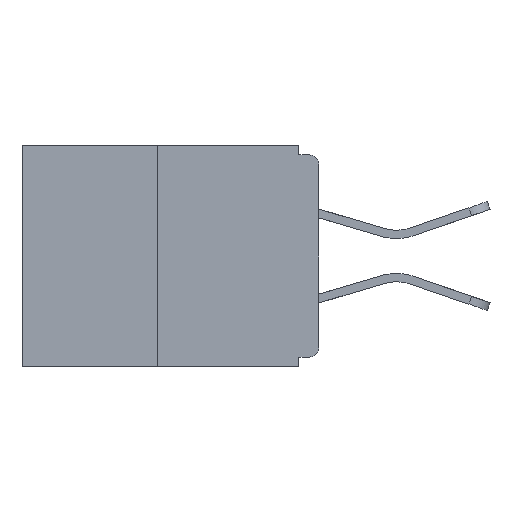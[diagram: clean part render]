
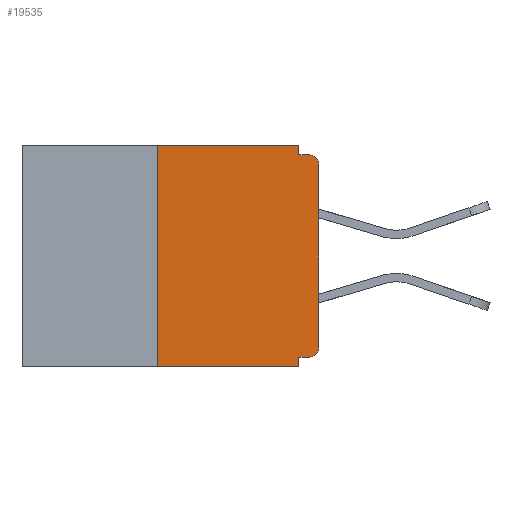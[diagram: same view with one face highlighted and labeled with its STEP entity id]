
A CAD part, left-side view. The second image highlights one B-rep face of the part: STEP entity #19535.
In plain terms, the highlighted planar face has unit normal (-1, 0, 0).
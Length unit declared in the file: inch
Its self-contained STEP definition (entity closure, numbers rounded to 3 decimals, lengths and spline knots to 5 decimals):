
#85 = CARTESIAN_POINT ( 'NONE',  ( 0., 0.015, -0.328 ) ) ;
#91 = LINE ( 'NONE', #1999, #10467 ) ;
#777 = LINE ( 'NONE', #20366, #14387 ) ;
#1901 = CARTESIAN_POINT ( 'NONE',  ( 0., 0., -0.313 ) ) ;
#1999 = CARTESIAN_POINT ( 'NONE',  ( 0., 0., -0.328 ) ) ;
#2536 = CARTESIAN_POINT ( 'NONE',  ( 0., 0.015, -0.015 ) ) ;
#2837 = AXIS2_PLACEMENT_3D ( 'NONE', #25909, #21193, #9138 ) ;
#2928 = DIRECTION ( 'NONE',  ( 0., -1., 0. ) ) ;
#3150 = CARTESIAN_POINT ( 'NONE',  ( 0., 0.031, -0.015 ) ) ;
#4056 = CARTESIAN_POINT ( 'NONE',  ( 0., 0.46, -0.343 ) ) ;
#4239 = DIRECTION ( 'NONE',  ( -1., 0., 0. ) ) ;
#4346 = CARTESIAN_POINT ( 'NONE',  ( 0., 0.015, -0.313 ) ) ;
#4563 = VERTEX_POINT ( 'NONE', #6031 ) ;
#4624 = ORIENTED_EDGE ( 'NONE', *, *, #10382, .F. ) ;
#5428 = EDGE_CURVE ( 'NONE', #14202, #19848, #8894, .T. ) ;
#5958 = EDGE_LOOP ( 'NONE', ( #14963, #21630, #27414, #29288, #4624, #13181, #27754, #19563, #12750, #11808 ) ) ;
#6020 = VECTOR ( 'NONE', #15183, 39.37008 ) ;
#6031 = CARTESIAN_POINT ( 'NONE',  ( 0., 0.25, 0. ) ) ;
#6893 = VERTEX_POINT ( 'NONE', #2536 ) ;
#7083 = VERTEX_POINT ( 'NONE', #10704 ) ;
#7120 = VERTEX_POINT ( 'NONE', #1901 ) ;
#7920 = DIRECTION ( 'NONE',  ( 0., 0., -1. ) ) ;
#8058 = EDGE_CURVE ( 'NONE', #12188, #31089, #14869, .T. ) ;
#8218 = CARTESIAN_POINT ( 'NONE',  ( 0., 0., 0. ) ) ;
#8294 = DIRECTION ( 'NONE',  ( 0., 0., -1. ) ) ;
#8894 = LINE ( 'NONE', #4056, #10368 ) ;
#9138 = DIRECTION ( 'NONE',  ( 0., 0., -1. ) ) ;
#9145 = EDGE_CURVE ( 'NONE', #4563, #12188, #777, .T. ) ;
#9616 = LINE ( 'NONE', #29054, #30650 ) ;
#10024 = CARTESIAN_POINT ( 'NONE',  ( 0., 0.031, -0.343 ) ) ;
#10355 = DIRECTION ( 'NONE',  ( 0., -1., 0. ) ) ;
#10368 = VECTOR ( 'NONE', #25677, 39.37008 ) ;
#10382 = EDGE_CURVE ( 'NONE', #16863, #7083, #91, .T. ) ;
#10456 = AXIS2_PLACEMENT_3D ( 'NONE', #13997, #4239, #21135 ) ;
#10467 = VECTOR ( 'NONE', #31000, 39.37008 ) ;
#10704 = CARTESIAN_POINT ( 'NONE',  ( 0., 0.031, -0.328 ) ) ;
#10972 = CIRCLE ( 'NONE', #10456, 0.015 ) ;
#11144 = AXIS2_PLACEMENT_3D ( 'NONE', #4346, #18560, #18248 ) ;
#11808 = ORIENTED_EDGE ( 'NONE', *, *, #8058, .F. ) ;
#12188 = VERTEX_POINT ( 'NONE', #18408 ) ;
#12449 = DIRECTION ( 'NONE',  ( 0., 0., 1. ) ) ;
#12750 = ORIENTED_EDGE ( 'NONE', *, *, #18966, .F. ) ;
#13181 = ORIENTED_EDGE ( 'NONE', *, *, #30544, .T. ) ;
#13997 = CARTESIAN_POINT ( 'NONE',  ( 0., 0.015, -0.03 ) ) ;
#14202 = VERTEX_POINT ( 'NONE', #30343 ) ;
#14387 = VECTOR ( 'NONE', #10355, 39.37008 ) ;
#14869 = LINE ( 'NONE', #29579, #15141 ) ;
#14963 = ORIENTED_EDGE ( 'NONE', *, *, #9145, .F. ) ;
#15141 = VECTOR ( 'NONE', #7920, 39.37008 ) ;
#15183 = DIRECTION ( 'NONE',  ( 0., 0., 1. ) ) ;
#15695 = CIRCLE ( 'NONE', #11144, 0.015 ) ;
#16863 = VERTEX_POINT ( 'NONE', #85 ) ;
#17106 = LINE ( 'NONE', #29758, #30547 ) ;
#17182 = CARTESIAN_POINT ( 'NONE',  ( 0., 0.031, -0.343 ) ) ;
#17781 = LINE ( 'NONE', #10024, #25567 ) ;
#18248 = DIRECTION ( 'NONE',  ( 0., 0., -1. ) ) ;
#18408 = CARTESIAN_POINT ( 'NONE',  ( 0., 0.031, 0. ) ) ;
#18503 = PLANE ( 'NONE',  #2837 ) ;
#18560 = DIRECTION ( 'NONE',  ( -1., 0., 0. ) ) ;
#18966 = EDGE_CURVE ( 'NONE', #31089, #6893, #17106, .T. ) ;
#19535 = ADVANCED_FACE ( 'NONE', ( #20732 ), #18503, .F. ) ;
#19563 = ORIENTED_EDGE ( 'NONE', *, *, #21149, .T. ) ;
#19773 = EDGE_CURVE ( 'NONE', #7083, #19848, #17781, .T. ) ;
#19848 = VERTEX_POINT ( 'NONE', #17182 ) ;
#20113 = LINE ( 'NONE', #8218, #6020 ) ;
#20366 = CARTESIAN_POINT ( 'NONE',  ( 0., 0.46, 0. ) ) ;
#20732 = FACE_OUTER_BOUND ( 'NONE', #5958, .T. ) ;
#21135 = DIRECTION ( 'NONE',  ( 0., 0., -1. ) ) ;
#21149 = EDGE_CURVE ( 'NONE', #30868, #6893, #10972, .T. ) ;
#21193 = DIRECTION ( 'NONE',  ( 1., 0., 0. ) ) ;
#21630 = ORIENTED_EDGE ( 'NONE', *, *, #28561, .F. ) ;
#25567 = VECTOR ( 'NONE', #8294, 39.37008 ) ;
#25677 = DIRECTION ( 'NONE',  ( 0., -1., 0. ) ) ;
#25909 = CARTESIAN_POINT ( 'NONE',  ( 0., 0.46, 0. ) ) ;
#27414 = ORIENTED_EDGE ( 'NONE', *, *, #5428, .T. ) ;
#27478 = CARTESIAN_POINT ( 'NONE',  ( 0., 0., -0.03 ) ) ;
#27754 = ORIENTED_EDGE ( 'NONE', *, *, #29515, .T. ) ;
#28561 = EDGE_CURVE ( 'NONE', #14202, #4563, #9616, .T. ) ;
#29054 = CARTESIAN_POINT ( 'NONE',  ( 0., 0.25, 0. ) ) ;
#29288 = ORIENTED_EDGE ( 'NONE', *, *, #19773, .F. ) ;
#29515 = EDGE_CURVE ( 'NONE', #7120, #30868, #20113, .T. ) ;
#29579 = CARTESIAN_POINT ( 'NONE',  ( 0., 0.031, 0. ) ) ;
#29758 = CARTESIAN_POINT ( 'NONE',  ( 0., 0., -0.015 ) ) ;
#30343 = CARTESIAN_POINT ( 'NONE',  ( 0., 0.25, -0.343 ) ) ;
#30544 = EDGE_CURVE ( 'NONE', #16863, #7120, #15695, .T. ) ;
#30547 = VECTOR ( 'NONE', #2928, 39.37008 ) ;
#30650 = VECTOR ( 'NONE', #12449, 39.37008 ) ;
#30868 = VERTEX_POINT ( 'NONE', #27478 ) ;
#31000 = DIRECTION ( 'NONE',  ( 0., 1., 0. ) ) ;
#31089 = VERTEX_POINT ( 'NONE', #3150 ) ;
